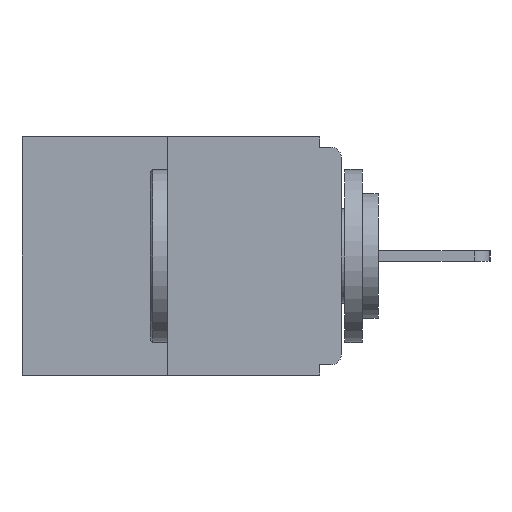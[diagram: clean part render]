
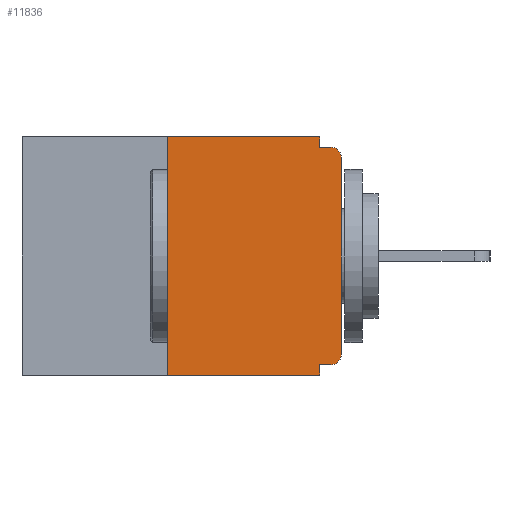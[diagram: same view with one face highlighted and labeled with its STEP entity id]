
A CAD part, left-side view. The second image highlights one B-rep face of the part: STEP entity #11836.
In plain terms, the highlighted planar face has unit normal (-1, 0, 0).
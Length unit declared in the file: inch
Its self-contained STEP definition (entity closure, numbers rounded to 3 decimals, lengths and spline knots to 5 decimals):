
#160 = DIRECTION ( 'NONE',  ( 0., 0., 1. ) ) ;
#175 = VECTOR ( 'NONE', #9141, 39.37008 ) ;
#381 = LINE ( 'NONE', #7069, #20362 ) ;
#709 = ORIENTED_EDGE ( 'NONE', *, *, #4707, .T. ) ;
#820 = FACE_OUTER_BOUND ( 'NONE', #12829, .T. ) ;
#847 = VERTEX_POINT ( 'NONE', #8901 ) ;
#916 = ORIENTED_EDGE ( 'NONE', *, *, #9475, .F. ) ;
#918 = CARTESIAN_POINT ( 'NONE',  ( 0., 0.015, -0.03 ) ) ;
#1594 = CARTESIAN_POINT ( 'NONE',  ( 0., 0.031, 0. ) ) ;
#2015 = VERTEX_POINT ( 'NONE', #9968 ) ;
#2105 = VERTEX_POINT ( 'NONE', #20624 ) ;
#2443 = DIRECTION ( 'NONE',  ( 0., -1., 0. ) ) ;
#2476 = ORIENTED_EDGE ( 'NONE', *, *, #11895, .T. ) ;
#2920 = AXIS2_PLACEMENT_3D ( 'NONE', #17396, #19059, #7590 ) ;
#3116 = CARTESIAN_POINT ( 'NONE',  ( 0., 0., 0. ) ) ;
#3199 = CIRCLE ( 'NONE', #11618, 0.015 ) ;
#3681 = CARTESIAN_POINT ( 'NONE',  ( 0., 0.015, -0.328 ) ) ;
#3968 = VERTEX_POINT ( 'NONE', #21637 ) ;
#4457 = DIRECTION ( 'NONE',  ( -1., 0., 0. ) ) ;
#4707 = EDGE_CURVE ( 'NONE', #7812, #2105, #3199, .T. ) ;
#5172 = DIRECTION ( 'NONE',  ( 0., 0., 1. ) ) ;
#6189 = VERTEX_POINT ( 'NONE', #6507 ) ;
#6372 = CARTESIAN_POINT ( 'NONE',  ( 0., 0., -0.03 ) ) ;
#6393 = ORIENTED_EDGE ( 'NONE', *, *, #15036, .F. ) ;
#6507 = CARTESIAN_POINT ( 'NONE',  ( 0., 0.25, -0.343 ) ) ;
#7069 = CARTESIAN_POINT ( 'NONE',  ( 0., 0.46, 0. ) ) ;
#7308 = CARTESIAN_POINT ( 'NONE',  ( 0., 0.015, -0.313 ) ) ;
#7405 = VECTOR ( 'NONE', #10719, 39.37008 ) ;
#7525 = CARTESIAN_POINT ( 'NONE',  ( 0., 0., -0.313 ) ) ;
#7581 = DIRECTION ( 'NONE',  ( -1., 0., 0. ) ) ;
#7590 = DIRECTION ( 'NONE',  ( 0., 0., -1. ) ) ;
#7647 = CARTESIAN_POINT ( 'NONE',  ( 0., 0.25, 0. ) ) ;
#7812 = VERTEX_POINT ( 'NONE', #6372 ) ;
#8176 = VECTOR ( 'NONE', #5172, 39.37008 ) ;
#8600 = LINE ( 'NONE', #18388, #13907 ) ;
#8819 = VERTEX_POINT ( 'NONE', #7647 ) ;
#8901 = CARTESIAN_POINT ( 'NONE',  ( 0., 0.031, -0.328 ) ) ;
#8950 = CARTESIAN_POINT ( 'NONE',  ( 0., 0.031, 0. ) ) ;
#9018 = DIRECTION ( 'NONE',  ( 0., -1., 0. ) ) ;
#9069 = EDGE_CURVE ( 'NONE', #6189, #3968, #17007, .T. ) ;
#9141 = DIRECTION ( 'NONE',  ( 0., 1., 0. ) ) ;
#9211 = ORIENTED_EDGE ( 'NONE', *, *, #9069, .T. ) ;
#9432 = EDGE_CURVE ( 'NONE', #2015, #2105, #12651, .T. ) ;
#9475 = EDGE_CURVE ( 'NONE', #847, #3968, #19041, .T. ) ;
#9706 = LINE ( 'NONE', #3116, #8176 ) ;
#9968 = CARTESIAN_POINT ( 'NONE',  ( 0., 0.031, -0.015 ) ) ;
#10639 = VECTOR ( 'NONE', #14977, 39.37008 ) ;
#10719 = DIRECTION ( 'NONE',  ( 0., -1., 0. ) ) ;
#10729 = VERTEX_POINT ( 'NONE', #3681 ) ;
#10829 = DIRECTION ( 'NONE',  ( 0., 0., -1. ) ) ;
#10903 = PLANE ( 'NONE',  #2920 ) ;
#11326 = CARTESIAN_POINT ( 'NONE',  ( 0., 0., -0.328 ) ) ;
#11600 = VERTEX_POINT ( 'NONE', #7525 ) ;
#11618 = AXIS2_PLACEMENT_3D ( 'NONE', #918, #7581, #14300 ) ;
#11836 = ADVANCED_FACE ( 'NONE', ( #820 ), #10903, .F. ) ;
#11895 = EDGE_CURVE ( 'NONE', #11600, #7812, #9706, .T. ) ;
#11910 = ORIENTED_EDGE ( 'NONE', *, *, #12038, .F. ) ;
#12038 = EDGE_CURVE ( 'NONE', #13090, #2015, #16645, .T. ) ;
#12651 = LINE ( 'NONE', #19371, #15858 ) ;
#12829 = EDGE_LOOP ( 'NONE', ( #15981, #6393, #9211, #916, #19652, #19994, #2476, #709, #18000, #11910 ) ) ;
#13090 = VERTEX_POINT ( 'NONE', #8950 ) ;
#13534 = EDGE_CURVE ( 'NONE', #10729, #847, #17401, .T. ) ;
#13907 = VECTOR ( 'NONE', #160, 39.37008 ) ;
#14300 = DIRECTION ( 'NONE',  ( 0., 0., -1. ) ) ;
#14362 = EDGE_CURVE ( 'NONE', #10729, #11600, #17384, .T. ) ;
#14597 = AXIS2_PLACEMENT_3D ( 'NONE', #7308, #4457, #10829 ) ;
#14977 = DIRECTION ( 'NONE',  ( 0., 0., -1. ) ) ;
#15036 = EDGE_CURVE ( 'NONE', #6189, #8819, #8600, .T. ) ;
#15344 = CARTESIAN_POINT ( 'NONE',  ( 0., 0.46, -0.343 ) ) ;
#15711 = CARTESIAN_POINT ( 'NONE',  ( 0., 0.031, -0.343 ) ) ;
#15858 = VECTOR ( 'NONE', #2443, 39.37008 ) ;
#15981 = ORIENTED_EDGE ( 'NONE', *, *, #18062, .F. ) ;
#16645 = LINE ( 'NONE', #1594, #10639 ) ;
#17007 = LINE ( 'NONE', #15344, #7405 ) ;
#17384 = CIRCLE ( 'NONE', #14597, 0.015 ) ;
#17396 = CARTESIAN_POINT ( 'NONE',  ( 0., 0.46, 0. ) ) ;
#17401 = LINE ( 'NONE', #11326, #175 ) ;
#18000 = ORIENTED_EDGE ( 'NONE', *, *, #9432, .F. ) ;
#18062 = EDGE_CURVE ( 'NONE', #8819, #13090, #381, .T. ) ;
#18388 = CARTESIAN_POINT ( 'NONE',  ( 0., 0.25, 0. ) ) ;
#19041 = LINE ( 'NONE', #15711, #20473 ) ;
#19059 = DIRECTION ( 'NONE',  ( 1., 0., 0. ) ) ;
#19371 = CARTESIAN_POINT ( 'NONE',  ( 0., 0., -0.015 ) ) ;
#19652 = ORIENTED_EDGE ( 'NONE', *, *, #13534, .F. ) ;
#19994 = ORIENTED_EDGE ( 'NONE', *, *, #14362, .T. ) ;
#20362 = VECTOR ( 'NONE', #9018, 39.37008 ) ;
#20473 = VECTOR ( 'NONE', #20811, 39.37008 ) ;
#20624 = CARTESIAN_POINT ( 'NONE',  ( 0., 0.015, -0.015 ) ) ;
#20811 = DIRECTION ( 'NONE',  ( 0., 0., -1. ) ) ;
#21637 = CARTESIAN_POINT ( 'NONE',  ( 0., 0.031, -0.343 ) ) ;
